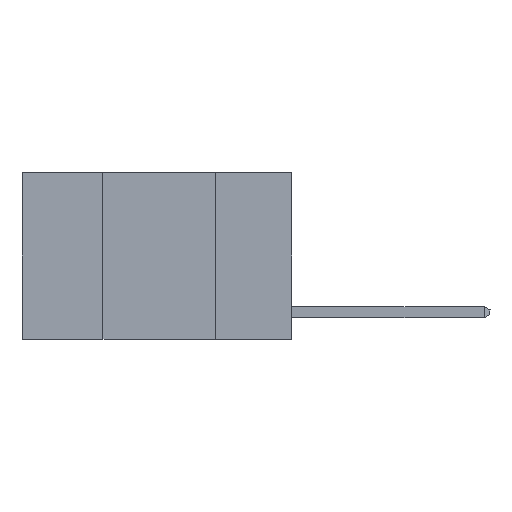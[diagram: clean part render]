
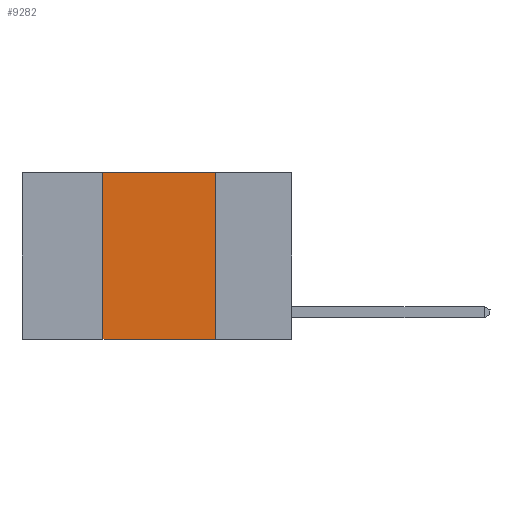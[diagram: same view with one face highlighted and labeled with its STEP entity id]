
A CAD part, left-side view. The second image highlights one B-rep face of the part: STEP entity #9282.
In plain terms, the highlighted planar face has unit normal (-1, 0, 0).
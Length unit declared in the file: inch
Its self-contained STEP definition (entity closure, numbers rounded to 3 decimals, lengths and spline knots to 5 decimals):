
#58 = CARTESIAN_POINT ( 'NONE',  ( 0., 0.6, 0. ) ) ;
#103 = VECTOR ( 'NONE', #17209, 39.37008 ) ;
#152 = VERTEX_POINT ( 'NONE', #8780 ) ;
#1036 = DIRECTION ( 'NONE',  ( 0., 0., -1. ) ) ;
#2344 = EDGE_CURVE ( 'NONE', #4177, #16976, #6667, .T. ) ;
#2735 = DIRECTION ( 'NONE',  ( 1., 0., 0. ) ) ;
#2794 = FACE_OUTER_BOUND ( 'NONE', #9476, .T. ) ;
#2917 = ORIENTED_EDGE ( 'NONE', *, *, #5656, .F. ) ;
#4177 = VERTEX_POINT ( 'NONE', #6672 ) ;
#5654 = CARTESIAN_POINT ( 'NONE',  ( 0., 0.17, 0. ) ) ;
#5656 = EDGE_CURVE ( 'NONE', #16976, #152, #17798, .T. ) ;
#5677 = ORIENTED_EDGE ( 'NONE', *, *, #20704, .F. ) ;
#6667 = LINE ( 'NONE', #18276, #16537 ) ;
#6672 = CARTESIAN_POINT ( 'NONE',  ( 0., 0.42, -0.37 ) ) ;
#7273 = EDGE_CURVE ( 'NONE', #4177, #17328, #19403, .T. ) ;
#8259 = CARTESIAN_POINT ( 'NONE',  ( 0., 0.6, -0.37 ) ) ;
#8780 = CARTESIAN_POINT ( 'NONE',  ( 0., 0.17, 0. ) ) ;
#9282 = ADVANCED_FACE ( 'NONE', ( #2794 ), #15203, .F. ) ;
#9476 = EDGE_LOOP ( 'NONE', ( #5677, #2917, #18828, #12995 ) ) ;
#10088 = LINE ( 'NONE', #5654, #21351 ) ;
#12303 = VECTOR ( 'NONE', #14083, 39.37008 ) ;
#12583 = CARTESIAN_POINT ( 'NONE',  ( 0., 0.42, 0. ) ) ;
#12775 = DIRECTION ( 'NONE',  ( 0., 0., -1. ) ) ;
#12995 = ORIENTED_EDGE ( 'NONE', *, *, #7273, .T. ) ;
#14083 = DIRECTION ( 'NONE',  ( 0., -1., 0. ) ) ;
#14887 = DIRECTION ( 'NONE',  ( 0., 0., 1. ) ) ;
#15203 = PLANE ( 'NONE',  #17855 ) ;
#16537 = VECTOR ( 'NONE', #14887, 39.37008 ) ;
#16976 = VERTEX_POINT ( 'NONE', #12583 ) ;
#17209 = DIRECTION ( 'NONE',  ( 0., -1., 0. ) ) ;
#17328 = VERTEX_POINT ( 'NONE', #17719 ) ;
#17719 = CARTESIAN_POINT ( 'NONE',  ( 0., 0.17, -0.37 ) ) ;
#17798 = LINE ( 'NONE', #58, #12303 ) ;
#17855 = AXIS2_PLACEMENT_3D ( 'NONE', #18642, #2735, #1036 ) ;
#18276 = CARTESIAN_POINT ( 'NONE',  ( 0., 0.42, 0. ) ) ;
#18642 = CARTESIAN_POINT ( 'NONE',  ( 0., 0.6, 0. ) ) ;
#18828 = ORIENTED_EDGE ( 'NONE', *, *, #2344, .F. ) ;
#19403 = LINE ( 'NONE', #8259, #103 ) ;
#20704 = EDGE_CURVE ( 'NONE', #152, #17328, #10088, .T. ) ;
#21351 = VECTOR ( 'NONE', #12775, 39.37008 ) ;
